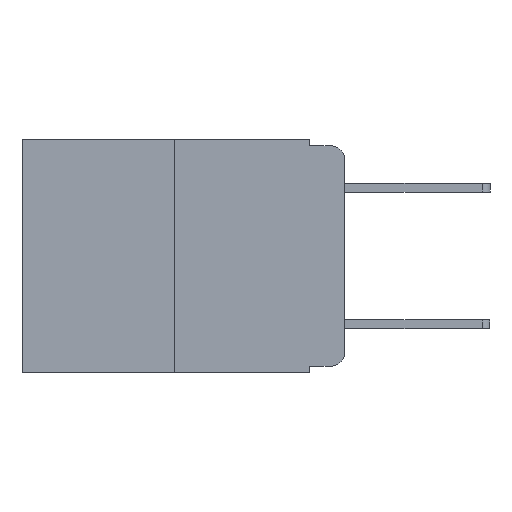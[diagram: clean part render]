
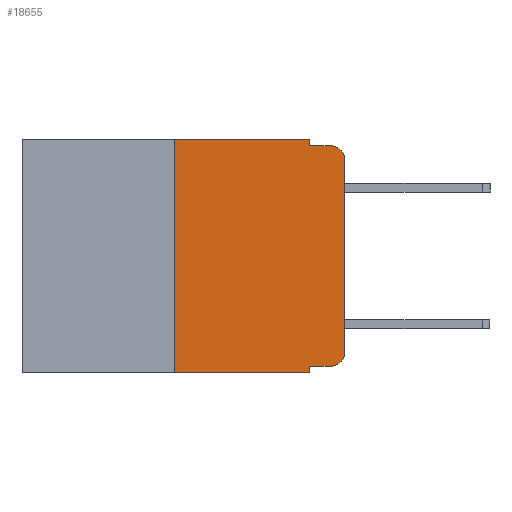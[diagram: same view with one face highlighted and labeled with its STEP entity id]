
A CAD part, left-side view. The second image highlights one B-rep face of the part: STEP entity #18655.
In plain terms, the highlighted planar face has unit normal (-1, 0, 0).
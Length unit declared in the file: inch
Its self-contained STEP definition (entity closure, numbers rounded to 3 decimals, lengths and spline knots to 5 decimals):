
#718 = DIRECTION ( 'NONE',  ( 0., -1., 0. ) ) ;
#778 = CARTESIAN_POINT ( 'NONE',  ( 0., 0.473, -0.343 ) ) ;
#826 = EDGE_CURVE ( 'NONE', #9545, #21196, #5144, .T. ) ;
#1022 = VERTEX_POINT ( 'NONE', #13374 ) ;
#1427 = LINE ( 'NONE', #2549, #20253 ) ;
#1568 = VECTOR ( 'NONE', #14831, 39.37008 ) ;
#2025 = CARTESIAN_POINT ( 'NONE',  ( 0., 0., 0. ) ) ;
#2110 = ORIENTED_EDGE ( 'NONE', *, *, #3837, .T. ) ;
#2215 = CARTESIAN_POINT ( 'NONE',  ( 0., 0.051, 0. ) ) ;
#2410 = ORIENTED_EDGE ( 'NONE', *, *, #18451, .F. ) ;
#2536 = DIRECTION ( 'NONE',  ( 0., 0., -1. ) ) ;
#2549 = CARTESIAN_POINT ( 'NONE',  ( 0., 0.051, -0.01 ) ) ;
#2863 = CARTESIAN_POINT ( 'NONE',  ( 0., 0.25, 0. ) ) ;
#3007 = ORIENTED_EDGE ( 'NONE', *, *, #16122, .T. ) ;
#3058 = DIRECTION ( 'NONE',  ( 0., 0., 1. ) ) ;
#3458 = EDGE_LOOP ( 'NONE', ( #3877, #18364, #9365, #10505, #20604, #2410, #3007, #8528, #4757, #2110 ) ) ;
#3690 = LINE ( 'NONE', #778, #8617 ) ;
#3837 = EDGE_CURVE ( 'NONE', #23141, #17751, #22764, .T. ) ;
#3877 = ORIENTED_EDGE ( 'NONE', *, *, #16832, .T. ) ;
#4007 = CARTESIAN_POINT ( 'NONE',  ( 0., 0.051, 0. ) ) ;
#4620 = EDGE_CURVE ( 'NONE', #21196, #20854, #1427, .T. ) ;
#4757 = ORIENTED_EDGE ( 'NONE', *, *, #11247, .T. ) ;
#4862 = LINE ( 'NONE', #15374, #22900 ) ;
#4963 = VECTOR ( 'NONE', #17718, 39.37008 ) ;
#5017 = CARTESIAN_POINT ( 'NONE',  ( 0., 0.473, 0. ) ) ;
#5144 = LINE ( 'NONE', #2215, #18478 ) ;
#5477 = CARTESIAN_POINT ( 'NONE',  ( 0., 0.473, 0. ) ) ;
#5696 = CARTESIAN_POINT ( 'NONE',  ( 0., 0.051, -0.343 ) ) ;
#7334 = DIRECTION ( 'NONE',  ( 1., 0., 0. ) ) ;
#8484 = FACE_OUTER_BOUND ( 'NONE', #3458, .T. ) ;
#8528 = ORIENTED_EDGE ( 'NONE', *, *, #16086, .F. ) ;
#8617 = VECTOR ( 'NONE', #11917, 39.37008 ) ;
#8776 = LINE ( 'NONE', #15872, #13621 ) ;
#8943 = DIRECTION ( 'NONE',  ( 0., -1., 0. ) ) ;
#9319 = DIRECTION ( 'NONE',  ( 0., 0., -1. ) ) ;
#9365 = ORIENTED_EDGE ( 'NONE', *, *, #4620, .F. ) ;
#9481 = VERTEX_POINT ( 'NONE', #5696 ) ;
#9493 = CARTESIAN_POINT ( 'NONE',  ( 0., 0.02, -0.333 ) ) ;
#9545 = VERTEX_POINT ( 'NONE', #4007 ) ;
#9873 = LINE ( 'NONE', #5017, #4963 ) ;
#10451 = DIRECTION ( 'NONE',  ( -1., 0., 0. ) ) ;
#10483 = EDGE_CURVE ( 'NONE', #16180, #9545, #9873, .T. ) ;
#10505 = ORIENTED_EDGE ( 'NONE', *, *, #826, .F. ) ;
#11247 = EDGE_CURVE ( 'NONE', #1022, #23141, #12437, .T. ) ;
#11875 = CARTESIAN_POINT ( 'NONE',  ( 0., 0.25, -0.343 ) ) ;
#11917 = DIRECTION ( 'NONE',  ( 0., -1., 0. ) ) ;
#12437 = LINE ( 'NONE', #19718, #13575 ) ;
#13374 = CARTESIAN_POINT ( 'NONE',  ( 0., 0.051, -0.333 ) ) ;
#13575 = VECTOR ( 'NONE', #8943, 39.37008 ) ;
#13621 = VECTOR ( 'NONE', #3058, 39.37008 ) ;
#14427 = EDGE_CURVE ( 'NONE', #19479, #20854, #15223, .T. ) ;
#14831 = DIRECTION ( 'NONE',  ( 0., 0., 1. ) ) ;
#15223 = CIRCLE ( 'NONE', #18290, 0.02 ) ;
#15374 = CARTESIAN_POINT ( 'NONE',  ( 0., 0.051, 0. ) ) ;
#15633 = AXIS2_PLACEMENT_3D ( 'NONE', #18331, #18225, #20364 ) ;
#15829 = CARTESIAN_POINT ( 'NONE',  ( 0., 0., -0.313 ) ) ;
#15872 = CARTESIAN_POINT ( 'NONE',  ( 0., 0.25, 0. ) ) ;
#16086 = EDGE_CURVE ( 'NONE', #1022, #9481, #4862, .T. ) ;
#16122 = EDGE_CURVE ( 'NONE', #22214, #9481, #3690, .T. ) ;
#16180 = VERTEX_POINT ( 'NONE', #2863 ) ;
#16234 = LINE ( 'NONE', #2025, #1568 ) ;
#16388 = PLANE ( 'NONE',  #21034 ) ;
#16832 = EDGE_CURVE ( 'NONE', #17751, #19479, #16234, .T. ) ;
#17718 = DIRECTION ( 'NONE',  ( 0., -1., 0. ) ) ;
#17751 = VERTEX_POINT ( 'NONE', #15829 ) ;
#18225 = DIRECTION ( 'NONE',  ( -1., 0., 0. ) ) ;
#18290 = AXIS2_PLACEMENT_3D ( 'NONE', #21169, #10451, #22929 ) ;
#18331 = CARTESIAN_POINT ( 'NONE',  ( 0., 0.02, -0.313 ) ) ;
#18364 = ORIENTED_EDGE ( 'NONE', *, *, #14427, .T. ) ;
#18451 = EDGE_CURVE ( 'NONE', #22214, #16180, #8776, .T. ) ;
#18478 = VECTOR ( 'NONE', #9319, 39.37008 ) ;
#18655 = ADVANCED_FACE ( 'NONE', ( #8484 ), #16388, .F. ) ;
#19479 = VERTEX_POINT ( 'NONE', #19902 ) ;
#19691 = CARTESIAN_POINT ( 'NONE',  ( 0., 0.02, -0.01 ) ) ;
#19718 = CARTESIAN_POINT ( 'NONE',  ( 0., 0.051, -0.333 ) ) ;
#19902 = CARTESIAN_POINT ( 'NONE',  ( 0., 0., -0.03 ) ) ;
#19952 = DIRECTION ( 'NONE',  ( 0., 0., -1. ) ) ;
#20253 = VECTOR ( 'NONE', #718, 39.37008 ) ;
#20364 = DIRECTION ( 'NONE',  ( 0., 0., -1. ) ) ;
#20604 = ORIENTED_EDGE ( 'NONE', *, *, #10483, .F. ) ;
#20751 = CARTESIAN_POINT ( 'NONE',  ( 0., 0.051, -0.01 ) ) ;
#20854 = VERTEX_POINT ( 'NONE', #19691 ) ;
#21034 = AXIS2_PLACEMENT_3D ( 'NONE', #5477, #7334, #19952 ) ;
#21169 = CARTESIAN_POINT ( 'NONE',  ( 0., 0.02, -0.03 ) ) ;
#21196 = VERTEX_POINT ( 'NONE', #20751 ) ;
#22214 = VERTEX_POINT ( 'NONE', #11875 ) ;
#22764 = CIRCLE ( 'NONE', #15633, 0.02 ) ;
#22900 = VECTOR ( 'NONE', #2536, 39.37008 ) ;
#22929 = DIRECTION ( 'NONE',  ( 0., 0., -1. ) ) ;
#23141 = VERTEX_POINT ( 'NONE', #9493 ) ;
